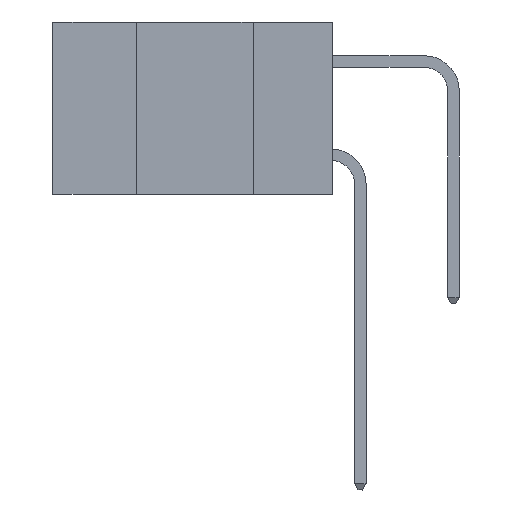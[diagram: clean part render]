
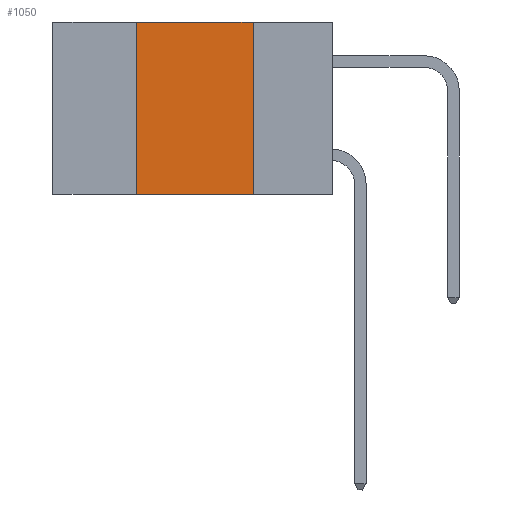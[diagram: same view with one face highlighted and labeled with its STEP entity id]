
A CAD part, left-side view. The second image highlights one B-rep face of the part: STEP entity #1050.
In plain terms, the highlighted planar face has unit normal (-1, 0, 0).
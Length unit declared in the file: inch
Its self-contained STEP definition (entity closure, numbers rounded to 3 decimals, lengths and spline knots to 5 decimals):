
#862 = VECTOR ( 'NONE', #9546, 39.37008 ) ;
#1050 = ADVANCED_FACE ( 'NONE', ( #7580 ), #3755, .F. ) ;
#1168 = VERTEX_POINT ( 'NONE', #6812 ) ;
#1630 = VERTEX_POINT ( 'NONE', #6737 ) ;
#2239 = VECTOR ( 'NONE', #2795, 39.37008 ) ;
#2795 = DIRECTION ( 'NONE',  ( 0., 0., -1. ) ) ;
#3069 = CARTESIAN_POINT ( 'NONE',  ( 0., 0.6, 0. ) ) ;
#3218 = ORIENTED_EDGE ( 'NONE', *, *, #10539, .F. ) ;
#3425 = VECTOR ( 'NONE', #12143, 39.37008 ) ;
#3754 = EDGE_CURVE ( 'NONE', #5523, #1168, #10170, .T. ) ;
#3755 = PLANE ( 'NONE',  #4473 ) ;
#3797 = LINE ( 'NONE', #6675, #3425 ) ;
#4062 = EDGE_LOOP ( 'NONE', ( #7084, #3218, #11913, #4168 ) ) ;
#4168 = ORIENTED_EDGE ( 'NONE', *, *, #4414, .T. ) ;
#4318 = EDGE_CURVE ( 'NONE', #1630, #6277, #13702, .T. ) ;
#4414 = EDGE_CURVE ( 'NONE', #5523, #6277, #3797, .T. ) ;
#4473 = AXIS2_PLACEMENT_3D ( 'NONE', #3069, #12719, #7004 ) ;
#5523 = VERTEX_POINT ( 'NONE', #11527 ) ;
#6277 = VERTEX_POINT ( 'NONE', #7972 ) ;
#6675 = CARTESIAN_POINT ( 'NONE',  ( 0., 0.6, -0.37 ) ) ;
#6737 = CARTESIAN_POINT ( 'NONE',  ( 0., 0.17, 0. ) ) ;
#6812 = CARTESIAN_POINT ( 'NONE',  ( 0., 0.42, 0. ) ) ;
#7004 = DIRECTION ( 'NONE',  ( 0., 0., -1. ) ) ;
#7084 = ORIENTED_EDGE ( 'NONE', *, *, #4318, .F. ) ;
#7580 = FACE_OUTER_BOUND ( 'NONE', #4062, .T. ) ;
#7972 = CARTESIAN_POINT ( 'NONE',  ( 0., 0.17, -0.37 ) ) ;
#9546 = DIRECTION ( 'NONE',  ( 0., -1., 0. ) ) ;
#10170 = LINE ( 'NONE', #10776, #13028 ) ;
#10539 = EDGE_CURVE ( 'NONE', #1168, #1630, #12807, .T. ) ;
#10772 = DIRECTION ( 'NONE',  ( 0., 0., 1. ) ) ;
#10776 = CARTESIAN_POINT ( 'NONE',  ( 0., 0.42, 0. ) ) ;
#11527 = CARTESIAN_POINT ( 'NONE',  ( 0., 0.42, -0.37 ) ) ;
#11913 = ORIENTED_EDGE ( 'NONE', *, *, #3754, .F. ) ;
#12143 = DIRECTION ( 'NONE',  ( 0., -1., 0. ) ) ;
#12719 = DIRECTION ( 'NONE',  ( 1., 0., 0. ) ) ;
#12807 = LINE ( 'NONE', #13852, #862 ) ;
#13028 = VECTOR ( 'NONE', #10772, 39.37008 ) ;
#13702 = LINE ( 'NONE', #14208, #2239 ) ;
#13852 = CARTESIAN_POINT ( 'NONE',  ( 0., 0.6, 0. ) ) ;
#14208 = CARTESIAN_POINT ( 'NONE',  ( 0., 0.17, 0. ) ) ;
